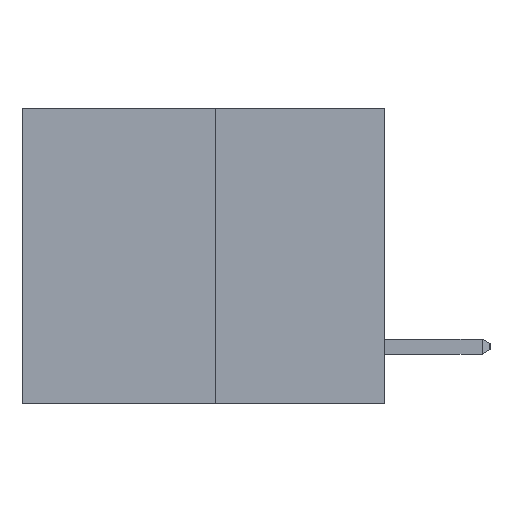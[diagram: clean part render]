
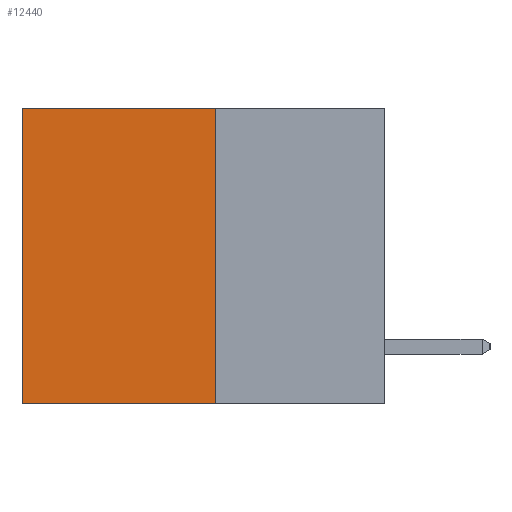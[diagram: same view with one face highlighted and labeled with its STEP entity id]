
A CAD part, left-side view. The second image highlights one B-rep face of the part: STEP entity #12440.
In plain terms, the highlighted planar face has unit normal (-1, 0, 0).
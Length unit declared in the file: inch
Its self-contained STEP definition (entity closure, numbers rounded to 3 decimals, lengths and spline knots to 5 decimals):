
#211 = DIRECTION ( 'NONE',  ( 0., 1., 0. ) ) ;
#1865 = LINE ( 'NONE', #12581, #4124 ) ;
#1899 = VECTOR ( 'NONE', #6587, 39.37008 ) ;
#1915 = CARTESIAN_POINT ( 'NONE',  ( 0.3165, 0.28, -0.49 ) ) ;
#2135 = LINE ( 'NONE', #6657, #1899 ) ;
#2565 = EDGE_LOOP ( 'NONE', ( #5882, #10633, #12965, #11160 ) ) ;
#2725 = CARTESIAN_POINT ( 'NONE',  ( 0.3165, 0.28, -0.49 ) ) ;
#3343 = VERTEX_POINT ( 'NONE', #16386 ) ;
#4124 = VECTOR ( 'NONE', #16888, 39.37008 ) ;
#4142 = FACE_OUTER_BOUND ( 'NONE', #2565, .T. ) ;
#4374 = DIRECTION ( 'NONE',  ( 0., 0., -1. ) ) ;
#5674 = VERTEX_POINT ( 'NONE', #1915 ) ;
#5882 = ORIENTED_EDGE ( 'NONE', *, *, #18668, .T. ) ;
#6587 = DIRECTION ( 'NONE',  ( 0., 1., 0. ) ) ;
#6657 = CARTESIAN_POINT ( 'NONE',  ( 0.3165, 0.28, -0.49 ) ) ;
#7210 = DIRECTION ( 'NONE',  ( 0., 0., -1. ) ) ;
#7279 = PLANE ( 'NONE',  #8742 ) ;
#8593 = LINE ( 'NONE', #2725, #15021 ) ;
#8742 = AXIS2_PLACEMENT_3D ( 'NONE', #10480, #15907, #7210 ) ;
#8802 = EDGE_CURVE ( 'NONE', #3343, #10755, #14588, .T. ) ;
#9079 = EDGE_CURVE ( 'NONE', #3343, #5674, #8593, .T. ) ;
#10480 = CARTESIAN_POINT ( 'NONE',  ( 0.3165, 0.28, -0.49 ) ) ;
#10633 = ORIENTED_EDGE ( 'NONE', *, *, #12129, .F. ) ;
#10755 = VERTEX_POINT ( 'NONE', #10901 ) ;
#10901 = CARTESIAN_POINT ( 'NONE',  ( 0.3165, 0.6, 0. ) ) ;
#11160 = ORIENTED_EDGE ( 'NONE', *, *, #8802, .T. ) ;
#12129 = EDGE_CURVE ( 'NONE', #5674, #14004, #2135, .T. ) ;
#12440 = ADVANCED_FACE ( 'NONE', ( #4142 ), #7279, .F. ) ;
#12581 = CARTESIAN_POINT ( 'NONE',  ( 0.3165, 0.6, -0.49 ) ) ;
#12965 = ORIENTED_EDGE ( 'NONE', *, *, #9079, .F. ) ;
#14004 = VERTEX_POINT ( 'NONE', #18909 ) ;
#14588 = LINE ( 'NONE', #14721, #17365 ) ;
#14721 = CARTESIAN_POINT ( 'NONE',  ( 0.3165, 0.28, 0. ) ) ;
#15021 = VECTOR ( 'NONE', #4374, 39.37008 ) ;
#15907 = DIRECTION ( 'NONE',  ( 1., 0., 0. ) ) ;
#16386 = CARTESIAN_POINT ( 'NONE',  ( 0.3165, 0.28, 0. ) ) ;
#16888 = DIRECTION ( 'NONE',  ( 0., 0., -1. ) ) ;
#17365 = VECTOR ( 'NONE', #211, 39.37008 ) ;
#18668 = EDGE_CURVE ( 'NONE', #10755, #14004, #1865, .T. ) ;
#18909 = CARTESIAN_POINT ( 'NONE',  ( 0.3165, 0.6, -0.49 ) ) ;
